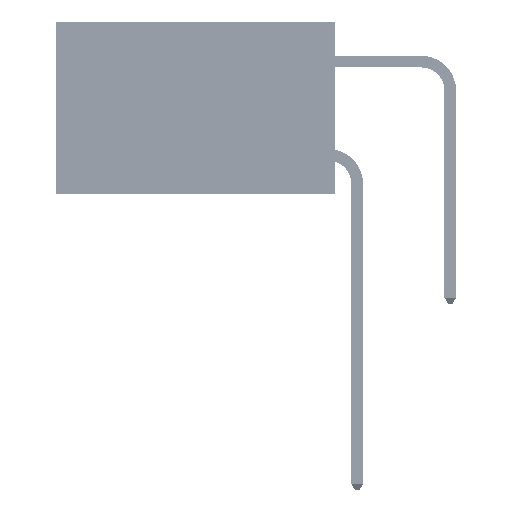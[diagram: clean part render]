
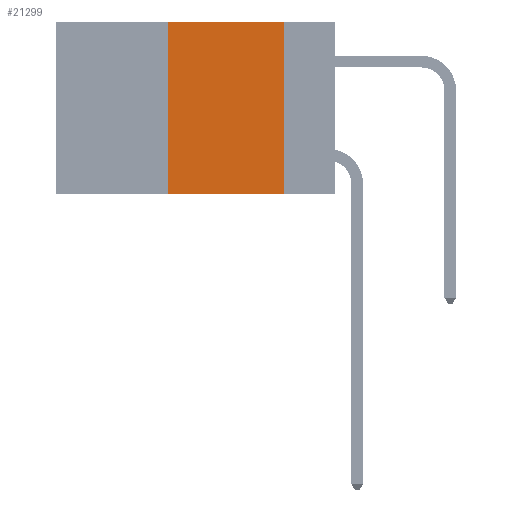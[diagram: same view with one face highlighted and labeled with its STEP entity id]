
A CAD part, left-side view. The second image highlights one B-rep face of the part: STEP entity #21299.
In plain terms, the highlighted planar face has unit normal (-1, 0, 0).
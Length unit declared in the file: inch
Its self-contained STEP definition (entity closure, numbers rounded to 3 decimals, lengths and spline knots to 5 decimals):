
#296 = LINE ( 'NONE', #33859, #9221 ) ;
#1277 = VERTEX_POINT ( 'NONE', #24292 ) ;
#3128 = DIRECTION ( 'NONE',  ( 0., 0., -1. ) ) ;
#3508 = ORIENTED_EDGE ( 'NONE', *, *, #29505, .F. ) ;
#4562 = CARTESIAN_POINT ( 'NONE',  ( 0., 0.11, 0. ) ) ;
#5244 = DIRECTION ( 'NONE',  ( 0., 0., -1. ) ) ;
#7273 = ORIENTED_EDGE ( 'NONE', *, *, #28273, .T. ) ;
#8193 = LINE ( 'NONE', #30143, #41646 ) ;
#9221 = VECTOR ( 'NONE', #26222, 39.37008 ) ;
#11627 = DIRECTION ( 'NONE',  ( 1., 0., 0. ) ) ;
#12538 = VECTOR ( 'NONE', #13490, 39.37008 ) ;
#12586 = VERTEX_POINT ( 'NONE', #15796 ) ;
#13490 = DIRECTION ( 'NONE',  ( 0., 0., 1. ) ) ;
#15352 = EDGE_CURVE ( 'NONE', #12586, #21322, #23306, .T. ) ;
#15796 = CARTESIAN_POINT ( 'NONE',  ( 0., 0.36, -0.37 ) ) ;
#21299 = ADVANCED_FACE ( 'NONE', ( #44243 ), #47650, .F. ) ;
#21322 = VERTEX_POINT ( 'NONE', #39678 ) ;
#23306 = LINE ( 'NONE', #34152, #12538 ) ;
#24292 = CARTESIAN_POINT ( 'NONE',  ( 0., 0.11, -0.37 ) ) ;
#26222 = DIRECTION ( 'NONE',  ( 0., -1., 0. ) ) ;
#27312 = CARTESIAN_POINT ( 'NONE',  ( 0., 0.6, 0. ) ) ;
#27785 = AXIS2_PLACEMENT_3D ( 'NONE', #27312, #11627, #3128 ) ;
#28263 = ORIENTED_EDGE ( 'NONE', *, *, #15352, .F. ) ;
#28273 = EDGE_CURVE ( 'NONE', #12586, #1277, #296, .T. ) ;
#28953 = CARTESIAN_POINT ( 'NONE',  ( 0., 0.11, 0. ) ) ;
#29505 = EDGE_CURVE ( 'NONE', #21322, #30688, #8193, .T. ) ;
#30143 = CARTESIAN_POINT ( 'NONE',  ( 0., 0.6, 0. ) ) ;
#30688 = VERTEX_POINT ( 'NONE', #28953 ) ;
#33859 = CARTESIAN_POINT ( 'NONE',  ( 0., 0.6, -0.37 ) ) ;
#34152 = CARTESIAN_POINT ( 'NONE',  ( 0., 0.36, 0. ) ) ;
#34370 = DIRECTION ( 'NONE',  ( 0., -1., 0. ) ) ;
#34541 = EDGE_LOOP ( 'NONE', ( #44853, #3508, #28263, #7273 ) ) ;
#37514 = VECTOR ( 'NONE', #5244, 39.37008 ) ;
#39678 = CARTESIAN_POINT ( 'NONE',  ( 0., 0.36, 0. ) ) ;
#40718 = LINE ( 'NONE', #4562, #37514 ) ;
#41646 = VECTOR ( 'NONE', #34370, 39.37008 ) ;
#44243 = FACE_OUTER_BOUND ( 'NONE', #34541, .T. ) ;
#44451 = EDGE_CURVE ( 'NONE', #30688, #1277, #40718, .T. ) ;
#44853 = ORIENTED_EDGE ( 'NONE', *, *, #44451, .F. ) ;
#47650 = PLANE ( 'NONE',  #27785 ) ;
